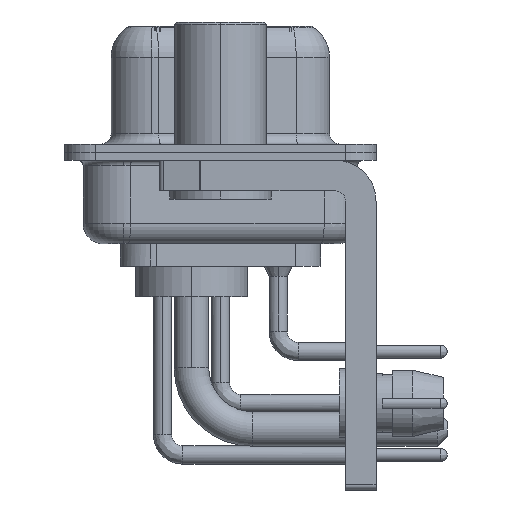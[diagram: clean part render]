
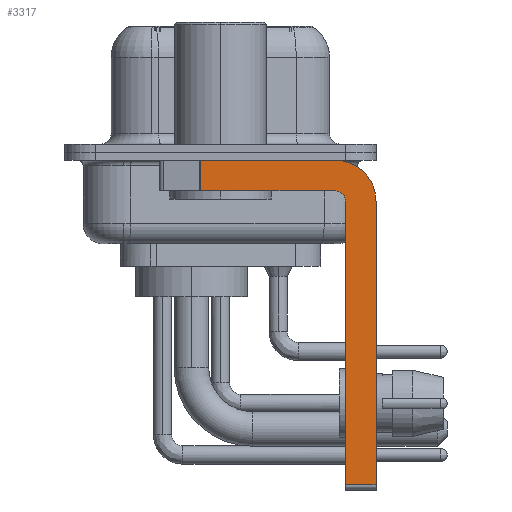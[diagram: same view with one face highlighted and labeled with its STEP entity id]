
A CAD part, left-side view. The second image highlights one B-rep face of the part: STEP entity #3317.
In plain terms, the highlighted planar face has unit normal (-1, 0, 0).
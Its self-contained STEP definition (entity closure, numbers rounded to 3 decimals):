
#319 = ORIENTED_EDGE ( 'NONE', *, *, #23579, .F. ) ;
#372 = LINE ( 'NONE', #9113, #18109 ) ;
#1118 = VERTEX_POINT ( 'NONE', #3757 ) ;
#1274 = CIRCLE ( 'NONE', #6142, 2. ) ;
#1705 = VERTEX_POINT ( 'NONE', #25633 ) ;
#2279 = EDGE_CURVE ( 'NONE', #1118, #27824, #30882, .T. ) ;
#2337 = CARTESIAN_POINT ( 'NONE',  ( -2.9, -5.65, -1.9 ) ) ;
#2461 = FACE_OUTER_BOUND ( 'NONE', #29163, .T. ) ;
#2650 = DIRECTION ( 'NONE',  ( 1., 0., 0. ) ) ;
#3028 = LINE ( 'NONE', #26342, #31754 ) ;
#3317 = ADVANCED_FACE ( 'NONE', ( #2461 ), #22915, .F. ) ;
#3662 = EDGE_CURVE ( 'NONE', #33272, #7305, #26896, .T. ) ;
#3757 = CARTESIAN_POINT ( 'NONE',  ( -2.9, -7.65, -2.4 ) ) ;
#3856 = ORIENTED_EDGE ( 'NONE', *, *, #14187, .F. ) ;
#4498 = CARTESIAN_POINT ( 'NONE',  ( -2.9, 0.978, -0.4 ) ) ;
#4590 = VERTEX_POINT ( 'NONE', #28626 ) ;
#4941 = CARTESIAN_POINT ( 'NONE',  ( -2.9, -7.65, -2.4 ) ) ;
#6142 = AXIS2_PLACEMENT_3D ( 'NONE', #8260, #34041, #30627 ) ;
#6683 = DIRECTION ( 'NONE',  ( 0., 0., 1. ) ) ;
#7281 = CARTESIAN_POINT ( 'NONE',  ( -2.9, -5.65, -2.4 ) ) ;
#7305 = VERTEX_POINT ( 'NONE', #24629 ) ;
#7476 = ORIENTED_EDGE ( 'NONE', *, *, #8371, .T. ) ;
#8017 = VECTOR ( 'NONE', #16489, 1000. ) ;
#8260 = CARTESIAN_POINT ( 'NONE',  ( -2.9, -5.65, -2.4 ) ) ;
#8371 = EDGE_CURVE ( 'NONE', #33272, #24981, #372, .T. ) ;
#9113 = CARTESIAN_POINT ( 'NONE',  ( -2.9, 0.978, -1.9 ) ) ;
#9540 = DIRECTION ( 'NONE',  ( 0., 0., 1. ) ) ;
#11187 = CARTESIAN_POINT ( 'NONE',  ( -2.9, -5.65, -2.4 ) ) ;
#11432 = EDGE_CURVE ( 'NONE', #7305, #1118, #1274, .T. ) ;
#12547 = LINE ( 'NONE', #29786, #19805 ) ;
#12977 = CIRCLE ( 'NONE', #37190, 0.5 ) ;
#14187 = EDGE_CURVE ( 'NONE', #1705, #4590, #12977, .T. ) ;
#14883 = VERTEX_POINT ( 'NONE', #23432 ) ;
#16489 = DIRECTION ( 'NONE',  ( 0., 0., -1. ) ) ;
#16564 = CARTESIAN_POINT ( 'NONE',  ( -2.9, 0.978, -1.9 ) ) ;
#17871 = ORIENTED_EDGE ( 'NONE', *, *, #23318, .F. ) ;
#18109 = VECTOR ( 'NONE', #20851, 1000. ) ;
#19805 = VECTOR ( 'NONE', #6683, 1000. ) ;
#20268 = DIRECTION ( 'NONE',  ( 0., -1., 0. ) ) ;
#20851 = DIRECTION ( 'NONE',  ( 0., 0., -1. ) ) ;
#21689 = VECTOR ( 'NONE', #32567, 1000. ) ;
#22915 = PLANE ( 'NONE',  #28278 ) ;
#23318 = EDGE_CURVE ( 'NONE', #4590, #24981, #28310, .T. ) ;
#23432 = CARTESIAN_POINT ( 'NONE',  ( -2.9, -6.15, -16.35 ) ) ;
#23579 = EDGE_CURVE ( 'NONE', #14883, #1705, #12547, .T. ) ;
#23641 = ORIENTED_EDGE ( 'NONE', *, *, #3662, .F. ) ;
#24097 = ORIENTED_EDGE ( 'NONE', *, *, #11432, .F. ) ;
#24519 = DIRECTION ( 'NONE',  ( -1., 0., 0. ) ) ;
#24629 = CARTESIAN_POINT ( 'NONE',  ( -2.9, -5.65, -0.4 ) ) ;
#24981 = VERTEX_POINT ( 'NONE', #16564 ) ;
#25590 = DIRECTION ( 'NONE',  ( 0., 0., -1. ) ) ;
#25633 = CARTESIAN_POINT ( 'NONE',  ( -2.9, -6.15, -2.4 ) ) ;
#26342 = CARTESIAN_POINT ( 'NONE',  ( -2.9, -5.65, -16.35 ) ) ;
#26896 = LINE ( 'NONE', #30281, #21689 ) ;
#27034 = ORIENTED_EDGE ( 'NONE', *, *, #2279, .F. ) ;
#27824 = VERTEX_POINT ( 'NONE', #35875 ) ;
#28278 = AXIS2_PLACEMENT_3D ( 'NONE', #11187, #2650, #25590 ) ;
#28310 = LINE ( 'NONE', #2337, #35523 ) ;
#28626 = CARTESIAN_POINT ( 'NONE',  ( -2.9, -5.65, -1.9 ) ) ;
#29032 = ORIENTED_EDGE ( 'NONE', *, *, #29629, .T. ) ;
#29163 = EDGE_LOOP ( 'NONE', ( #23641, #7476, #17871, #3856, #319, #29032, #27034, #24097 ) ) ;
#29629 = EDGE_CURVE ( 'NONE', #14883, #27824, #3028, .T. ) ;
#29786 = CARTESIAN_POINT ( 'NONE',  ( -2.9, -6.15, -16.6 ) ) ;
#30281 = CARTESIAN_POINT ( 'NONE',  ( -2.9, 3., -0.4 ) ) ;
#30627 = DIRECTION ( 'NONE',  ( 0., 0., -1. ) ) ;
#30882 = LINE ( 'NONE', #4941, #8017 ) ;
#31754 = VECTOR ( 'NONE', #20268, 1000. ) ;
#32567 = DIRECTION ( 'NONE',  ( 0., -1., 0. ) ) ;
#33272 = VERTEX_POINT ( 'NONE', #4498 ) ;
#34041 = DIRECTION ( 'NONE',  ( 1., 0., 0. ) ) ;
#35523 = VECTOR ( 'NONE', #36667, 1000. ) ;
#35875 = CARTESIAN_POINT ( 'NONE',  ( -2.9, -7.65, -16.35 ) ) ;
#36667 = DIRECTION ( 'NONE',  ( 0., 1., 0. ) ) ;
#37190 = AXIS2_PLACEMENT_3D ( 'NONE', #7281, #24519, #9540 ) ;
